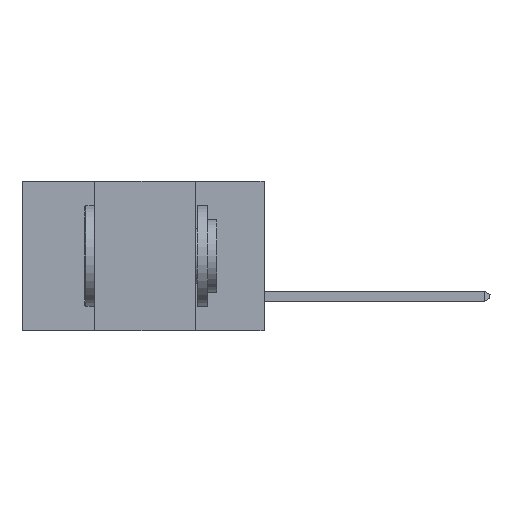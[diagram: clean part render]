
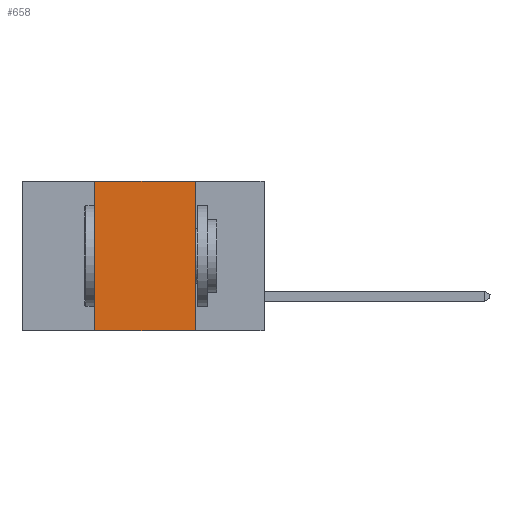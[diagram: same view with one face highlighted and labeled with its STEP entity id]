
A CAD part, left-side view. The second image highlights one B-rep face of the part: STEP entity #658.
In plain terms, the highlighted planar face has unit normal (-1, 0, 0).
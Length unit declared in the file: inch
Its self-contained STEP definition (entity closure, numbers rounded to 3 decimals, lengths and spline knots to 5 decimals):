
#658 = ADVANCED_FACE ( 'NONE', ( #9651 ), #26238, .F. ) ;
#1440 = CARTESIAN_POINT ( 'NONE',  ( 0., 0.6, 0. ) ) ;
#2297 = CARTESIAN_POINT ( 'NONE',  ( 0., 0.6, -0.37 ) ) ;
#3487 = LINE ( 'NONE', #14775, #22444 ) ;
#3957 = EDGE_CURVE ( 'NONE', #22164, #11225, #28810, .T. ) ;
#5673 = VECTOR ( 'NONE', #23713, 39.37008 ) ;
#6288 = AXIS2_PLACEMENT_3D ( 'NONE', #1440, #31914, #29146 ) ;
#7663 = DIRECTION ( 'NONE',  ( 0., 0., 1. ) ) ;
#9285 = VECTOR ( 'NONE', #29111, 39.37008 ) ;
#9651 = FACE_OUTER_BOUND ( 'NONE', #14954, .T. ) ;
#9669 = EDGE_CURVE ( 'NONE', #11225, #11678, #11861, .T. ) ;
#10393 = EDGE_CURVE ( 'NONE', #30240, #11678, #11837, .T. ) ;
#10816 = CARTESIAN_POINT ( 'NONE',  ( 0., 0.17, -0.37 ) ) ;
#11225 = VERTEX_POINT ( 'NONE', #12922 ) ;
#11678 = VERTEX_POINT ( 'NONE', #10816 ) ;
#11837 = LINE ( 'NONE', #2297, #5673 ) ;
#11861 = LINE ( 'NONE', #28896, #9285 ) ;
#12922 = CARTESIAN_POINT ( 'NONE',  ( 0., 0.17, 0. ) ) ;
#13302 = ORIENTED_EDGE ( 'NONE', *, *, #10393, .T. ) ;
#13459 = EDGE_CURVE ( 'NONE', #30240, #22164, #3487, .T. ) ;
#14178 = CARTESIAN_POINT ( 'NONE',  ( 0., 0.42, -0.37 ) ) ;
#14775 = CARTESIAN_POINT ( 'NONE',  ( 0., 0.42, 0. ) ) ;
#14954 = EDGE_LOOP ( 'NONE', ( #26218, #30695, #30842, #13302 ) ) ;
#21420 = VECTOR ( 'NONE', #24093, 39.37008 ) ;
#21593 = CARTESIAN_POINT ( 'NONE',  ( 0., 0.6, 0. ) ) ;
#22164 = VERTEX_POINT ( 'NONE', #24288 ) ;
#22444 = VECTOR ( 'NONE', #7663, 39.37008 ) ;
#23713 = DIRECTION ( 'NONE',  ( 0., -1., 0. ) ) ;
#24093 = DIRECTION ( 'NONE',  ( 0., -1., 0. ) ) ;
#24288 = CARTESIAN_POINT ( 'NONE',  ( 0., 0.42, 0. ) ) ;
#26218 = ORIENTED_EDGE ( 'NONE', *, *, #9669, .F. ) ;
#26238 = PLANE ( 'NONE',  #6288 ) ;
#28810 = LINE ( 'NONE', #21593, #21420 ) ;
#28896 = CARTESIAN_POINT ( 'NONE',  ( 0., 0.17, 0. ) ) ;
#29111 = DIRECTION ( 'NONE',  ( 0., 0., -1. ) ) ;
#29146 = DIRECTION ( 'NONE',  ( 0., 0., -1. ) ) ;
#30240 = VERTEX_POINT ( 'NONE', #14178 ) ;
#30695 = ORIENTED_EDGE ( 'NONE', *, *, #3957, .F. ) ;
#30842 = ORIENTED_EDGE ( 'NONE', *, *, #13459, .F. ) ;
#31914 = DIRECTION ( 'NONE',  ( 1., 0., 0. ) ) ;
